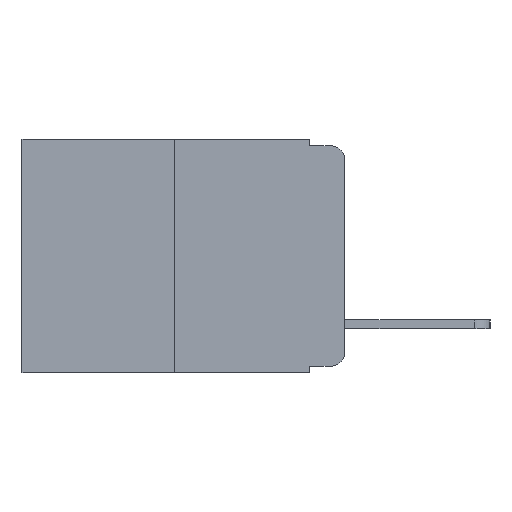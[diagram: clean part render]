
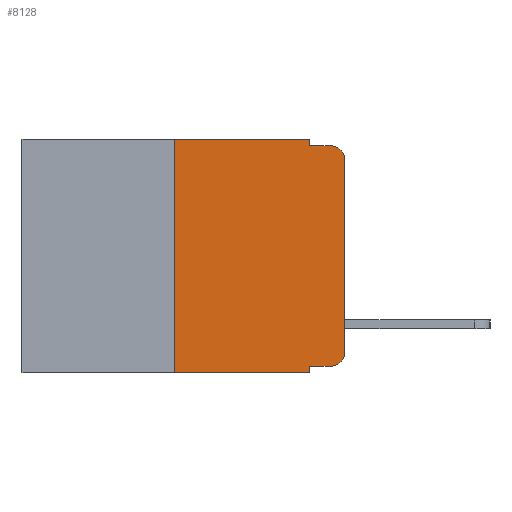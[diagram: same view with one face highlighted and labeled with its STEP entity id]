
A CAD part, left-side view. The second image highlights one B-rep face of the part: STEP entity #8128.
In plain terms, the highlighted planar face has unit normal (-1, 0, 0).
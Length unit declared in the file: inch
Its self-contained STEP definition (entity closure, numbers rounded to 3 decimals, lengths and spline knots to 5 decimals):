
#316 = AXIS2_PLACEMENT_3D ( 'NONE', #11700, #3619, #13009 ) ;
#335 = VERTEX_POINT ( 'NONE', #11621 ) ;
#480 = DIRECTION ( 'NONE',  ( 0., 0., -1. ) ) ;
#677 = ORIENTED_EDGE ( 'NONE', *, *, #5629, .F. ) ;
#712 = VERTEX_POINT ( 'NONE', #15805 ) ;
#804 = EDGE_LOOP ( 'NONE', ( #2268, #12987, #5634, #8159, #14800, #2570, #7438, #677, #4267, #14869 ) ) ;
#1481 = CARTESIAN_POINT ( 'NONE',  ( 0., 0.473, -0.343 ) ) ;
#1496 = LINE ( 'NONE', #15944, #4617 ) ;
#1776 = CARTESIAN_POINT ( 'NONE',  ( 0., 0.473, 0. ) ) ;
#1792 = EDGE_CURVE ( 'NONE', #9901, #7519, #13106, .T. ) ;
#2266 = LINE ( 'NONE', #12158, #5401 ) ;
#2268 = ORIENTED_EDGE ( 'NONE', *, *, #7225, .T. ) ;
#2508 = LINE ( 'NONE', #13278, #16191 ) ;
#2536 = DIRECTION ( 'NONE',  ( 0., -1., 0. ) ) ;
#2570 = ORIENTED_EDGE ( 'NONE', *, *, #1792, .F. ) ;
#2818 = DIRECTION ( 'NONE',  ( 0., -1., 0. ) ) ;
#2910 = AXIS2_PLACEMENT_3D ( 'NONE', #1776, #8536, #480 ) ;
#2917 = DIRECTION ( 'NONE',  ( 0., 0., -1. ) ) ;
#3486 = LINE ( 'NONE', #6966, #17078 ) ;
#3619 = DIRECTION ( 'NONE',  ( -1., 0., 0. ) ) ;
#3791 = DIRECTION ( 'NONE',  ( -1., 0., 0. ) ) ;
#3987 = VERTEX_POINT ( 'NONE', #11235 ) ;
#4052 = VERTEX_POINT ( 'NONE', #6008 ) ;
#4267 = ORIENTED_EDGE ( 'NONE', *, *, #11090, .T. ) ;
#4617 = VECTOR ( 'NONE', #10827, 39.37008 ) ;
#5401 = VECTOR ( 'NONE', #8139, 39.37008 ) ;
#5534 = VECTOR ( 'NONE', #10332, 39.37008 ) ;
#5629 = EDGE_CURVE ( 'NONE', #13376, #4052, #3486, .T. ) ;
#5634 = ORIENTED_EDGE ( 'NONE', *, *, #9876, .F. ) ;
#6008 = CARTESIAN_POINT ( 'NONE',  ( 0., 0.051, -0.343 ) ) ;
#6118 = VERTEX_POINT ( 'NONE', #13285 ) ;
#6917 = CARTESIAN_POINT ( 'NONE',  ( 0., 0.25, 0. ) ) ;
#6966 = CARTESIAN_POINT ( 'NONE',  ( 0., 0.051, 0. ) ) ;
#6968 = CARTESIAN_POINT ( 'NONE',  ( 0., 0.02, -0.333 ) ) ;
#7204 = PLANE ( 'NONE',  #2910 ) ;
#7225 = EDGE_CURVE ( 'NONE', #3987, #10707, #14113, .T. ) ;
#7438 = ORIENTED_EDGE ( 'NONE', *, *, #8618, .T. ) ;
#7519 = VERTEX_POINT ( 'NONE', #6917 ) ;
#8128 = ADVANCED_FACE ( 'NONE', ( #10596 ), #7204, .F. ) ;
#8139 = DIRECTION ( 'NONE',  ( 0., -1., 0. ) ) ;
#8159 = ORIENTED_EDGE ( 'NONE', *, *, #11195, .F. ) ;
#8536 = DIRECTION ( 'NONE',  ( 1., 0., 0. ) ) ;
#8618 = EDGE_CURVE ( 'NONE', #9901, #4052, #16610, .T. ) ;
#9056 = CIRCLE ( 'NONE', #316, 0.02 ) ;
#9144 = AXIS2_PLACEMENT_3D ( 'NONE', #11864, #3791, #13171 ) ;
#9320 = EDGE_CURVE ( 'NONE', #7519, #335, #1496, .T. ) ;
#9672 = DIRECTION ( 'NONE',  ( 0., 0., -1. ) ) ;
#9715 = EDGE_CURVE ( 'NONE', #14248, #3987, #9056, .T. ) ;
#9876 = EDGE_CURVE ( 'NONE', #712, #6118, #2508, .T. ) ;
#9901 = VERTEX_POINT ( 'NONE', #12030 ) ;
#10332 = DIRECTION ( 'NONE',  ( 0., 0., 1. ) ) ;
#10367 = CARTESIAN_POINT ( 'NONE',  ( 0., 0.051, -0.333 ) ) ;
#10596 = FACE_OUTER_BOUND ( 'NONE', #804, .T. ) ;
#10707 = VERTEX_POINT ( 'NONE', #11085 ) ;
#10827 = DIRECTION ( 'NONE',  ( 0., -1., 0. ) ) ;
#10918 = VECTOR ( 'NONE', #2917, 39.37008 ) ;
#11085 = CARTESIAN_POINT ( 'NONE',  ( 0., 0., -0.03 ) ) ;
#11090 = EDGE_CURVE ( 'NONE', #13376, #14248, #2266, .T. ) ;
#11195 = EDGE_CURVE ( 'NONE', #335, #712, #14378, .T. ) ;
#11235 = CARTESIAN_POINT ( 'NONE',  ( 0., 0., -0.313 ) ) ;
#11617 = EDGE_CURVE ( 'NONE', #10707, #6118, #12557, .T. ) ;
#11621 = CARTESIAN_POINT ( 'NONE',  ( 0., 0.051, 0. ) ) ;
#11667 = CARTESIAN_POINT ( 'NONE',  ( 0., 0., 0. ) ) ;
#11700 = CARTESIAN_POINT ( 'NONE',  ( 0., 0.02, -0.313 ) ) ;
#11864 = CARTESIAN_POINT ( 'NONE',  ( 0., 0.02, -0.03 ) ) ;
#12030 = CARTESIAN_POINT ( 'NONE',  ( 0., 0.25, -0.343 ) ) ;
#12158 = CARTESIAN_POINT ( 'NONE',  ( 0., 0.051, -0.333 ) ) ;
#12557 = CIRCLE ( 'NONE', #9144, 0.02 ) ;
#12987 = ORIENTED_EDGE ( 'NONE', *, *, #11617, .T. ) ;
#13009 = DIRECTION ( 'NONE',  ( 0., 0., -1. ) ) ;
#13106 = LINE ( 'NONE', #15194, #5534 ) ;
#13171 = DIRECTION ( 'NONE',  ( 0., 0., -1. ) ) ;
#13278 = CARTESIAN_POINT ( 'NONE',  ( 0., 0.051, -0.01 ) ) ;
#13285 = CARTESIAN_POINT ( 'NONE',  ( 0., 0.02, -0.01 ) ) ;
#13376 = VERTEX_POINT ( 'NONE', #10367 ) ;
#13635 = CARTESIAN_POINT ( 'NONE',  ( 0., 0.051, 0. ) ) ;
#13664 = VECTOR ( 'NONE', #2818, 39.37008 ) ;
#14113 = LINE ( 'NONE', #11667, #14501 ) ;
#14248 = VERTEX_POINT ( 'NONE', #6968 ) ;
#14307 = DIRECTION ( 'NONE',  ( 0., 0., 1. ) ) ;
#14378 = LINE ( 'NONE', #13635, #10918 ) ;
#14501 = VECTOR ( 'NONE', #14307, 39.37008 ) ;
#14800 = ORIENTED_EDGE ( 'NONE', *, *, #9320, .F. ) ;
#14869 = ORIENTED_EDGE ( 'NONE', *, *, #9715, .T. ) ;
#15194 = CARTESIAN_POINT ( 'NONE',  ( 0., 0.25, 0. ) ) ;
#15805 = CARTESIAN_POINT ( 'NONE',  ( 0., 0.051, -0.01 ) ) ;
#15944 = CARTESIAN_POINT ( 'NONE',  ( 0., 0.473, 0. ) ) ;
#16191 = VECTOR ( 'NONE', #2536, 39.37008 ) ;
#16610 = LINE ( 'NONE', #1481, #13664 ) ;
#17078 = VECTOR ( 'NONE', #9672, 39.37008 ) ;
